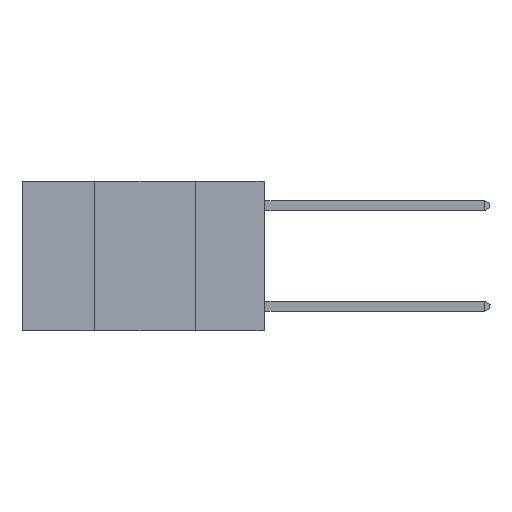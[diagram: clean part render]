
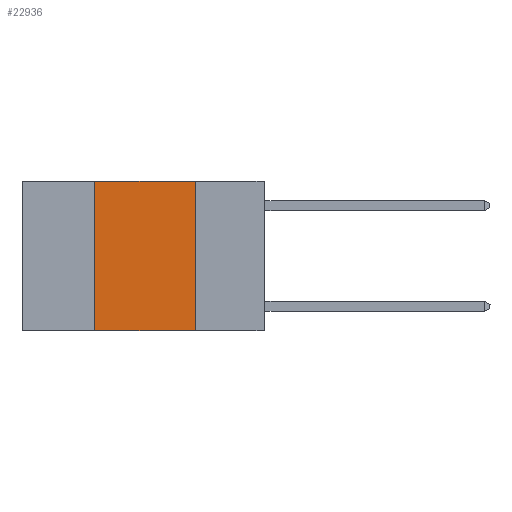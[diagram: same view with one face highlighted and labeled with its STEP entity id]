
A CAD part, left-side view. The second image highlights one B-rep face of the part: STEP entity #22936.
In plain terms, the highlighted planar face has unit normal (-1, 0, 0).
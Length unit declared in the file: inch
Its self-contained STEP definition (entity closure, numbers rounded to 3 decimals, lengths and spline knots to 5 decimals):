
#2270 = CARTESIAN_POINT ( 'NONE',  ( 0., 0.42, 0. ) ) ;
#2673 = CARTESIAN_POINT ( 'NONE',  ( 0., 0.17, -0.37 ) ) ;
#2679 = VERTEX_POINT ( 'NONE', #20677 ) ;
#3539 = FACE_OUTER_BOUND ( 'NONE', #29445, .T. ) ;
#3548 = EDGE_CURVE ( 'NONE', #28106, #2679, #25487, .T. ) ;
#3754 = VECTOR ( 'NONE', #21794, 39.37008 ) ;
#3872 = AXIS2_PLACEMENT_3D ( 'NONE', #28328, #13830, #30749 ) ;
#5541 = ORIENTED_EDGE ( 'NONE', *, *, #29566, .F. ) ;
#7289 = CARTESIAN_POINT ( 'NONE',  ( 0., 0.42, 0. ) ) ;
#7589 = ORIENTED_EDGE ( 'NONE', *, *, #30137, .F. ) ;
#7783 = LINE ( 'NONE', #19230, #18617 ) ;
#8905 = ORIENTED_EDGE ( 'NONE', *, *, #17627, .T. ) ;
#9062 = CARTESIAN_POINT ( 'NONE',  ( 0., 0.6, 0. ) ) ;
#10962 = VECTOR ( 'NONE', #29254, 39.37008 ) ;
#11604 = DIRECTION ( 'NONE',  ( 0., -1., 0. ) ) ;
#13830 = DIRECTION ( 'NONE',  ( 1., 0., 0. ) ) ;
#15207 = VECTOR ( 'NONE', #11604, 39.37008 ) ;
#17505 = LINE ( 'NONE', #2270, #10962 ) ;
#17627 = EDGE_CURVE ( 'NONE', #17872, #27449, #29030, .T. ) ;
#17872 = VERTEX_POINT ( 'NONE', #27514 ) ;
#18617 = VECTOR ( 'NONE', #26482, 39.37008 ) ;
#19230 = CARTESIAN_POINT ( 'NONE',  ( 0., 0.17, 0. ) ) ;
#20677 = CARTESIAN_POINT ( 'NONE',  ( 0., 0.17, 0. ) ) ;
#21129 = PLANE ( 'NONE',  #3872 ) ;
#21794 = DIRECTION ( 'NONE',  ( 0., -1., 0. ) ) ;
#22936 = ADVANCED_FACE ( 'NONE', ( #3539 ), #21129, .F. ) ;
#24058 = ORIENTED_EDGE ( 'NONE', *, *, #3548, .F. ) ;
#25487 = LINE ( 'NONE', #9062, #15207 ) ;
#26482 = DIRECTION ( 'NONE',  ( 0., 0., -1. ) ) ;
#26598 = CARTESIAN_POINT ( 'NONE',  ( 0., 0.6, -0.37 ) ) ;
#27449 = VERTEX_POINT ( 'NONE', #2673 ) ;
#27514 = CARTESIAN_POINT ( 'NONE',  ( 0., 0.42, -0.37 ) ) ;
#28106 = VERTEX_POINT ( 'NONE', #7289 ) ;
#28328 = CARTESIAN_POINT ( 'NONE',  ( 0., 0.6, 0. ) ) ;
#29030 = LINE ( 'NONE', #26598, #3754 ) ;
#29254 = DIRECTION ( 'NONE',  ( 0., 0., 1. ) ) ;
#29445 = EDGE_LOOP ( 'NONE', ( #7589, #24058, #5541, #8905 ) ) ;
#29566 = EDGE_CURVE ( 'NONE', #17872, #28106, #17505, .T. ) ;
#30137 = EDGE_CURVE ( 'NONE', #2679, #27449, #7783, .T. ) ;
#30749 = DIRECTION ( 'NONE',  ( 0., 0., -1. ) ) ;
